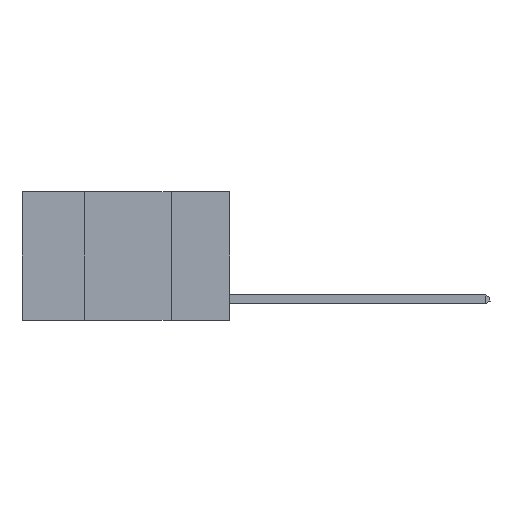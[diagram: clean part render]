
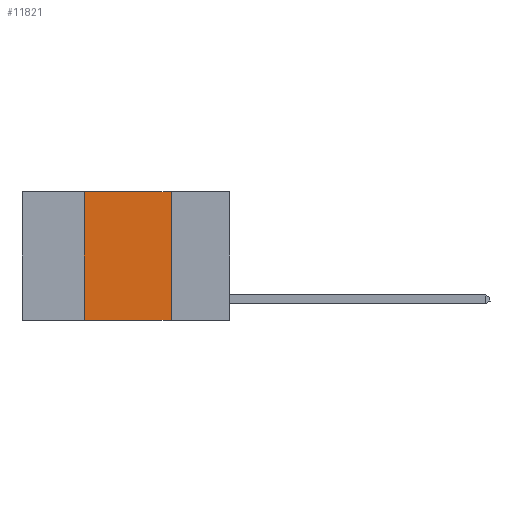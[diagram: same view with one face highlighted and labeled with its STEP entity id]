
A CAD part, left-side view. The second image highlights one B-rep face of the part: STEP entity #11821.
In plain terms, the highlighted planar face has unit normal (-1, 0, 0).
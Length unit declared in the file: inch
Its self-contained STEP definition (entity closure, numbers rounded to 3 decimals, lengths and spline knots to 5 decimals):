
#1179 = CARTESIAN_POINT ( 'NONE',  ( 0., 0.42, -0.37 ) ) ;
#1399 = AXIS2_PLACEMENT_3D ( 'NONE', #8140, #9442, #5531 ) ;
#1679 = LINE ( 'NONE', #16679, #8231 ) ;
#1743 = EDGE_CURVE ( 'NONE', #2717, #8216, #1679, .T. ) ;
#2157 = LINE ( 'NONE', #4629, #6787 ) ;
#2666 = FACE_OUTER_BOUND ( 'NONE', #6599, .T. ) ;
#2717 = VERTEX_POINT ( 'NONE', #5347 ) ;
#4374 = VECTOR ( 'NONE', #13860, 39.37008 ) ;
#4629 = CARTESIAN_POINT ( 'NONE',  ( 0., 0.42, 0. ) ) ;
#5347 = CARTESIAN_POINT ( 'NONE',  ( 0., 0.42, 0. ) ) ;
#5531 = DIRECTION ( 'NONE',  ( 0., 0., -1. ) ) ;
#5624 = LINE ( 'NONE', #16156, #4374 ) ;
#6513 = VERTEX_POINT ( 'NONE', #1179 ) ;
#6599 = EDGE_LOOP ( 'NONE', ( #10800, #11209, #17508, #7324 ) ) ;
#6787 = VECTOR ( 'NONE', #10263, 39.37008 ) ;
#7067 = CARTESIAN_POINT ( 'NONE',  ( 0., 0.17, 0. ) ) ;
#7324 = ORIENTED_EDGE ( 'NONE', *, *, #16951, .T. ) ;
#7796 = CARTESIAN_POINT ( 'NONE',  ( 0., 0.6, -0.37 ) ) ;
#8140 = CARTESIAN_POINT ( 'NONE',  ( 0., 0.6, 0. ) ) ;
#8216 = VERTEX_POINT ( 'NONE', #7067 ) ;
#8231 = VECTOR ( 'NONE', #11132, 39.37008 ) ;
#8870 = VERTEX_POINT ( 'NONE', #11307 ) ;
#9199 = PLANE ( 'NONE',  #1399 ) ;
#9384 = LINE ( 'NONE', #7796, #10917 ) ;
#9442 = DIRECTION ( 'NONE',  ( 1., 0., 0. ) ) ;
#10263 = DIRECTION ( 'NONE',  ( 0., 0., 1. ) ) ;
#10380 = EDGE_CURVE ( 'NONE', #6513, #2717, #2157, .T. ) ;
#10800 = ORIENTED_EDGE ( 'NONE', *, *, #17436, .F. ) ;
#10917 = VECTOR ( 'NONE', #13240, 39.37008 ) ;
#11132 = DIRECTION ( 'NONE',  ( 0., -1., 0. ) ) ;
#11209 = ORIENTED_EDGE ( 'NONE', *, *, #1743, .F. ) ;
#11307 = CARTESIAN_POINT ( 'NONE',  ( 0., 0.17, -0.37 ) ) ;
#11821 = ADVANCED_FACE ( 'NONE', ( #2666 ), #9199, .F. ) ;
#13240 = DIRECTION ( 'NONE',  ( 0., -1., 0. ) ) ;
#13860 = DIRECTION ( 'NONE',  ( 0., 0., -1. ) ) ;
#16156 = CARTESIAN_POINT ( 'NONE',  ( 0., 0.17, 0. ) ) ;
#16679 = CARTESIAN_POINT ( 'NONE',  ( 0., 0.6, 0. ) ) ;
#16951 = EDGE_CURVE ( 'NONE', #6513, #8870, #9384, .T. ) ;
#17436 = EDGE_CURVE ( 'NONE', #8216, #8870, #5624, .T. ) ;
#17508 = ORIENTED_EDGE ( 'NONE', *, *, #10380, .F. ) ;
